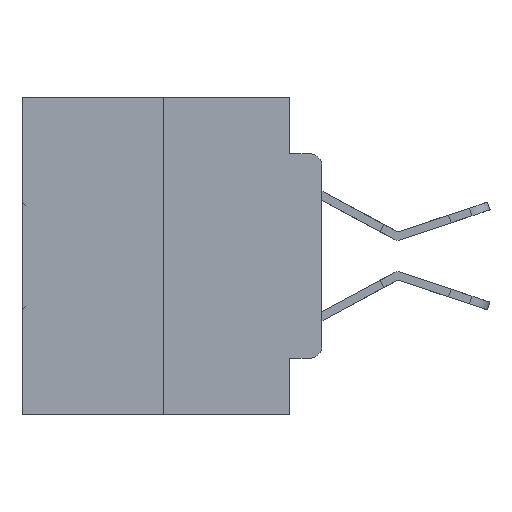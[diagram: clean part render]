
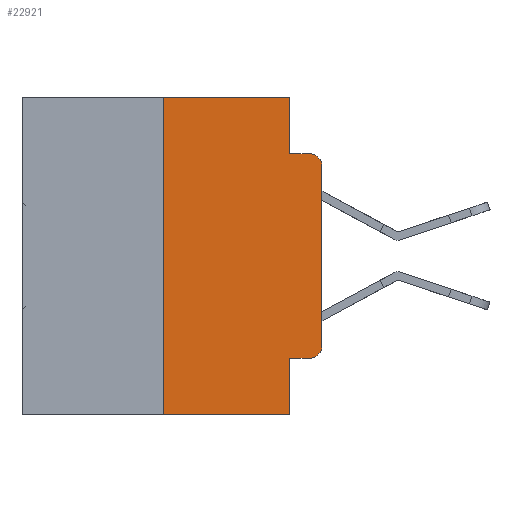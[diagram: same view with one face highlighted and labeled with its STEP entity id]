
A CAD part, left-side view. The second image highlights one B-rep face of the part: STEP entity #22921.
In plain terms, the highlighted planar face has unit normal (-1, 0, 0).
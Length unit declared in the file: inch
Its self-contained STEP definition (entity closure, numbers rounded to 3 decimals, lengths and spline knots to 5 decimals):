
#643 = DIRECTION ( 'NONE',  ( 0., 0., 1. ) ) ;
#941 = ORIENTED_EDGE ( 'NONE', *, *, #20094, .T. ) ;
#1186 = CARTESIAN_POINT ( 'NONE',  ( 0., 0.051, -0.0885 ) ) ;
#1400 = ORIENTED_EDGE ( 'NONE', *, *, #4757, .T. ) ;
#1426 = EDGE_CURVE ( 'NONE', #18013, #22416, #27641, .T. ) ;
#1682 = ORIENTED_EDGE ( 'NONE', *, *, #28006, .F. ) ;
#1780 = DIRECTION ( 'NONE',  ( 0., 0., -1. ) ) ;
#1867 = VERTEX_POINT ( 'NONE', #1936 ) ;
#1936 = CARTESIAN_POINT ( 'NONE',  ( 0., 0., -0.1085 ) ) ;
#2013 = LINE ( 'NONE', #17812, #8589 ) ;
#2110 = CARTESIAN_POINT ( 'NONE',  ( 0., 0.02, -0.4115 ) ) ;
#2474 = LINE ( 'NONE', #16476, #28219 ) ;
#2653 = VECTOR ( 'NONE', #22975, 39.37008 ) ;
#2922 = CARTESIAN_POINT ( 'NONE',  ( 0., 0.02, -0.1085 ) ) ;
#2954 = DIRECTION ( 'NONE',  ( -1., 0., 0. ) ) ;
#3087 = EDGE_CURVE ( 'NONE', #1867, #22416, #29729, .T. ) ;
#3229 = CARTESIAN_POINT ( 'NONE',  ( 0., 0.473, 0. ) ) ;
#3720 = ORIENTED_EDGE ( 'NONE', *, *, #23262, .T. ) ;
#3798 = CARTESIAN_POINT ( 'NONE',  ( 0., 0.051, 0. ) ) ;
#4624 = DIRECTION ( 'NONE',  ( 0., -1., 0. ) ) ;
#4757 = EDGE_CURVE ( 'NONE', #16427, #1867, #2013, .T. ) ;
#4827 = ORIENTED_EDGE ( 'NONE', *, *, #8169, .F. ) ;
#5484 = VECTOR ( 'NONE', #4624, 39.37008 ) ;
#5717 = DIRECTION ( 'NONE',  ( 0., 0., -1. ) ) ;
#5777 = VECTOR ( 'NONE', #23975, 39.37008 ) ;
#6030 = ORIENTED_EDGE ( 'NONE', *, *, #1426, .F. ) ;
#6504 = LINE ( 'NONE', #23955, #25095 ) ;
#6529 = DIRECTION ( 'NONE',  ( 0., 0., -1. ) ) ;
#6546 = LINE ( 'NONE', #11844, #5777 ) ;
#7432 = FACE_OUTER_BOUND ( 'NONE', #23120, .T. ) ;
#7937 = ORIENTED_EDGE ( 'NONE', *, *, #16407, .T. ) ;
#8169 = EDGE_CURVE ( 'NONE', #15465, #8267, #12077, .T. ) ;
#8267 = VERTEX_POINT ( 'NONE', #3798 ) ;
#8326 = CARTESIAN_POINT ( 'NONE',  ( 0., 0.25, 0. ) ) ;
#8366 = DIRECTION ( 'NONE',  ( 0., -1., 0. ) ) ;
#8475 = CARTESIAN_POINT ( 'NONE',  ( 0., 0.25, -0.5 ) ) ;
#8589 = VECTOR ( 'NONE', #643, 39.37008 ) ;
#9486 = DIRECTION ( 'NONE',  ( 0., -1., 0. ) ) ;
#10487 = CARTESIAN_POINT ( 'NONE',  ( 0., 0.02, -0.3915 ) ) ;
#11332 = CARTESIAN_POINT ( 'NONE',  ( 0., 0.02, -0.0885 ) ) ;
#11844 = CARTESIAN_POINT ( 'NONE',  ( 0., 0.25, 0. ) ) ;
#12077 = LINE ( 'NONE', #22848, #22643 ) ;
#12126 = ORIENTED_EDGE ( 'NONE', *, *, #24884, .F. ) ;
#12944 = DIRECTION ( 'NONE',  ( 0., 0., -1. ) ) ;
#13020 = ORIENTED_EDGE ( 'NONE', *, *, #31183, .F. ) ;
#14945 = VERTEX_POINT ( 'NONE', #15891 ) ;
#15465 = VERTEX_POINT ( 'NONE', #8326 ) ;
#15721 = CARTESIAN_POINT ( 'NONE',  ( 0., 0.051, 0. ) ) ;
#15891 = CARTESIAN_POINT ( 'NONE',  ( 0., 0.051, -0.5 ) ) ;
#16407 = EDGE_CURVE ( 'NONE', #21461, #14945, #6504, .T. ) ;
#16427 = VERTEX_POINT ( 'NONE', #16832 ) ;
#16476 = CARTESIAN_POINT ( 'NONE',  ( 0., 0.051, 0. ) ) ;
#16832 = CARTESIAN_POINT ( 'NONE',  ( 0., 0., -0.3915 ) ) ;
#17113 = DIRECTION ( 'NONE',  ( 0., -1., 0. ) ) ;
#17812 = CARTESIAN_POINT ( 'NONE',  ( 0., 0., 0. ) ) ;
#18013 = VERTEX_POINT ( 'NONE', #1186 ) ;
#18785 = VERTEX_POINT ( 'NONE', #30722 ) ;
#18865 = VERTEX_POINT ( 'NONE', #2110 ) ;
#20094 = EDGE_CURVE ( 'NONE', #18865, #16427, #25773, .T. ) ;
#20319 = DIRECTION ( 'NONE',  ( 1., 0., 0. ) ) ;
#21344 = VECTOR ( 'NONE', #17113, 39.37008 ) ;
#21461 = VERTEX_POINT ( 'NONE', #8475 ) ;
#21620 = ORIENTED_EDGE ( 'NONE', *, *, #3087, .T. ) ;
#22416 = VERTEX_POINT ( 'NONE', #11332 ) ;
#22643 = VECTOR ( 'NONE', #8366, 39.37008 ) ;
#22848 = CARTESIAN_POINT ( 'NONE',  ( 0., 0.473, 0. ) ) ;
#22921 = ADVANCED_FACE ( 'NONE', ( #7432 ), #25026, .F. ) ;
#22975 = DIRECTION ( 'NONE',  ( 0., 0., -1. ) ) ;
#23120 = EDGE_LOOP ( 'NONE', ( #1400, #21620, #6030, #13020, #4827, #1682, #7937, #12126, #3720, #941 ) ) ;
#23262 = EDGE_CURVE ( 'NONE', #18785, #18865, #29613, .T. ) ;
#23955 = CARTESIAN_POINT ( 'NONE',  ( 0., 0.473, -0.5 ) ) ;
#23975 = DIRECTION ( 'NONE',  ( 0., 0., 1. ) ) ;
#24062 = CARTESIAN_POINT ( 'NONE',  ( 0., 0.051, -0.4115 ) ) ;
#24884 = EDGE_CURVE ( 'NONE', #18785, #14945, #28400, .T. ) ;
#25026 = PLANE ( 'NONE',  #30730 ) ;
#25095 = VECTOR ( 'NONE', #9486, 39.37008 ) ;
#25648 = CARTESIAN_POINT ( 'NONE',  ( 0., 0.051, -0.0885 ) ) ;
#25773 = CIRCLE ( 'NONE', #27200, 0.02 ) ;
#27200 = AXIS2_PLACEMENT_3D ( 'NONE', #10487, #27289, #12944 ) ;
#27289 = DIRECTION ( 'NONE',  ( -1., 0., 0. ) ) ;
#27641 = LINE ( 'NONE', #25648, #21344 ) ;
#28006 = EDGE_CURVE ( 'NONE', #21461, #15465, #6546, .T. ) ;
#28219 = VECTOR ( 'NONE', #1780, 39.37008 ) ;
#28400 = LINE ( 'NONE', #15721, #2653 ) ;
#29061 = AXIS2_PLACEMENT_3D ( 'NONE', #2922, #2954, #6529 ) ;
#29613 = LINE ( 'NONE', #24062, #5484 ) ;
#29729 = CIRCLE ( 'NONE', #29061, 0.02 ) ;
#30722 = CARTESIAN_POINT ( 'NONE',  ( 0., 0.051, -0.4115 ) ) ;
#30730 = AXIS2_PLACEMENT_3D ( 'NONE', #3229, #20319, #5717 ) ;
#31183 = EDGE_CURVE ( 'NONE', #8267, #18013, #2474, .T. ) ;
